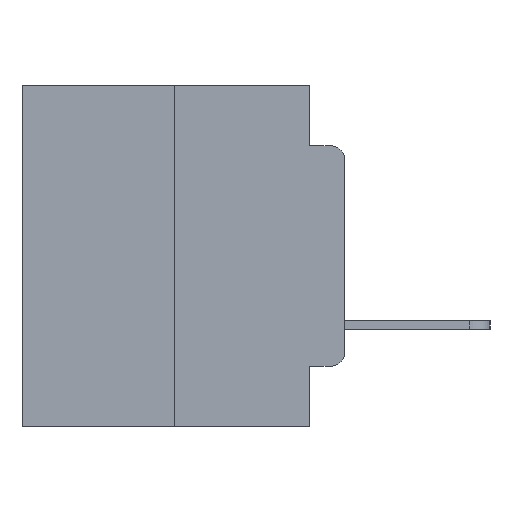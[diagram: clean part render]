
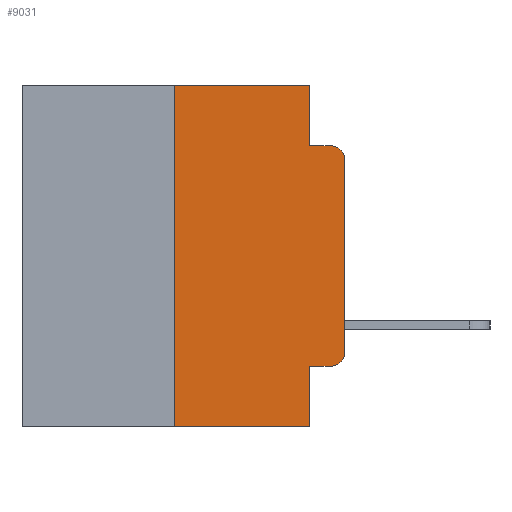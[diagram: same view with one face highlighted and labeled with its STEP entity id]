
A CAD part, left-side view. The second image highlights one B-rep face of the part: STEP entity #9031.
In plain terms, the highlighted planar face has unit normal (-1, 0, 0).
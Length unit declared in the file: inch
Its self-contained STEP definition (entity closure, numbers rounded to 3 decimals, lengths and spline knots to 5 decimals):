
#978 = DIRECTION ( 'NONE',  ( 1., 0., 0. ) ) ;
#1343 = ORIENTED_EDGE ( 'NONE', *, *, #14991, .T. ) ;
#1379 = ORIENTED_EDGE ( 'NONE', *, *, #8385, .F. ) ;
#1432 = ORIENTED_EDGE ( 'NONE', *, *, #3981, .F. ) ;
#1718 = CARTESIAN_POINT ( 'NONE',  ( 0., 0.473, 0. ) ) ;
#2085 = LINE ( 'NONE', #13930, #7773 ) ;
#2167 = PLANE ( 'NONE',  #11923 ) ;
#3199 = ORIENTED_EDGE ( 'NONE', *, *, #7303, .T. ) ;
#3981 = EDGE_CURVE ( 'NONE', #24997, #15552, #4936, .T. ) ;
#4006 = CARTESIAN_POINT ( 'NONE',  ( 0., 0.051, -0.0885 ) ) ;
#4120 = CARTESIAN_POINT ( 'NONE',  ( 0., 0.473, -0.5 ) ) ;
#4145 = CIRCLE ( 'NONE', #16932, 0.02 ) ;
#4783 = ORIENTED_EDGE ( 'NONE', *, *, #8187, .F. ) ;
#4809 = DIRECTION ( 'NONE',  ( 0., 0., -1. ) ) ;
#4936 = LINE ( 'NONE', #8817, #14816 ) ;
#5304 = VECTOR ( 'NONE', #20444, 39.37008 ) ;
#5547 = VERTEX_POINT ( 'NONE', #21693 ) ;
#5571 = FACE_OUTER_BOUND ( 'NONE', #15620, .T. ) ;
#5613 = VERTEX_POINT ( 'NONE', #19469 ) ;
#5883 = CARTESIAN_POINT ( 'NONE',  ( 0., 0., -0.1085 ) ) ;
#6039 = VECTOR ( 'NONE', #6686, 39.37008 ) ;
#6062 = VECTOR ( 'NONE', #9578, 39.37008 ) ;
#6412 = ORIENTED_EDGE ( 'NONE', *, *, #8388, .T. ) ;
#6423 = DIRECTION ( 'NONE',  ( 0., 0., -1. ) ) ;
#6652 = DIRECTION ( 'NONE',  ( 0., -1., 0. ) ) ;
#6680 = DIRECTION ( 'NONE',  ( -1., 0., 0. ) ) ;
#6686 = DIRECTION ( 'NONE',  ( 0., 0., -1. ) ) ;
#6707 = CARTESIAN_POINT ( 'NONE',  ( 0., 0.051, -0.4115 ) ) ;
#6713 = LINE ( 'NONE', #6707, #26224 ) ;
#6737 = CARTESIAN_POINT ( 'NONE',  ( 0., 0.051, 0. ) ) ;
#6741 = CARTESIAN_POINT ( 'NONE',  ( 0., 0.02, -0.1085 ) ) ;
#7303 = EDGE_CURVE ( 'NONE', #12543, #11504, #21738, .T. ) ;
#7340 = EDGE_CURVE ( 'NONE', #11504, #5547, #4145, .T. ) ;
#7463 = EDGE_CURVE ( 'NONE', #13498, #5547, #12701, .T. ) ;
#7526 = ORIENTED_EDGE ( 'NONE', *, *, #8641, .T. ) ;
#7773 = VECTOR ( 'NONE', #14446, 39.37008 ) ;
#8112 = EDGE_CURVE ( 'NONE', #15552, #13498, #2085, .T. ) ;
#8187 = EDGE_CURVE ( 'NONE', #5613, #24997, #16811, .T. ) ;
#8385 = EDGE_CURVE ( 'NONE', #17269, #15461, #22303, .T. ) ;
#8388 = EDGE_CURVE ( 'NONE', #17269, #11099, #6713, .T. ) ;
#8641 = EDGE_CURVE ( 'NONE', #11099, #12543, #20171, .T. ) ;
#8817 = CARTESIAN_POINT ( 'NONE',  ( 0., 0.473, 0. ) ) ;
#9031 = ADVANCED_FACE ( 'NONE', ( #5571 ), #2167, .F. ) ;
#9181 = CARTESIAN_POINT ( 'NONE',  ( 0., 0.051, -0.4115 ) ) ;
#9578 = DIRECTION ( 'NONE',  ( 0., 0., 1. ) ) ;
#9769 = CARTESIAN_POINT ( 'NONE',  ( 0., 0., 0. ) ) ;
#11099 = VERTEX_POINT ( 'NONE', #19550 ) ;
#11504 = VERTEX_POINT ( 'NONE', #5883 ) ;
#11923 = AXIS2_PLACEMENT_3D ( 'NONE', #1718, #978, #12239 ) ;
#12067 = VECTOR ( 'NONE', #12161, 39.37008 ) ;
#12161 = DIRECTION ( 'NONE',  ( 0., 0., 1. ) ) ;
#12193 = CARTESIAN_POINT ( 'NONE',  ( 0., 0.25, 0. ) ) ;
#12239 = DIRECTION ( 'NONE',  ( 0., 0., -1. ) ) ;
#12543 = VERTEX_POINT ( 'NONE', #19851 ) ;
#12701 = LINE ( 'NONE', #26269, #17400 ) ;
#13498 = VERTEX_POINT ( 'NONE', #4006 ) ;
#13930 = CARTESIAN_POINT ( 'NONE',  ( 0., 0.051, 0. ) ) ;
#14123 = CARTESIAN_POINT ( 'NONE',  ( 0., 0.051, 0. ) ) ;
#14446 = DIRECTION ( 'NONE',  ( 0., 0., -1. ) ) ;
#14816 = VECTOR ( 'NONE', #23032, 39.37008 ) ;
#14991 = EDGE_CURVE ( 'NONE', #5613, #15461, #16427, .T. ) ;
#15461 = VERTEX_POINT ( 'NONE', #23623 ) ;
#15552 = VERTEX_POINT ( 'NONE', #14123 ) ;
#15620 = EDGE_LOOP ( 'NONE', ( #3199, #19325, #25422, #26311, #1432, #4783, #1343, #1379, #6412, #7526 ) ) ;
#16427 = LINE ( 'NONE', #4120, #5304 ) ;
#16811 = LINE ( 'NONE', #12193, #12067 ) ;
#16932 = AXIS2_PLACEMENT_3D ( 'NONE', #6741, #6680, #6423 ) ;
#17269 = VERTEX_POINT ( 'NONE', #9181 ) ;
#17400 = VECTOR ( 'NONE', #26222, 39.37008 ) ;
#17450 = AXIS2_PLACEMENT_3D ( 'NONE', #23006, #23091, #4809 ) ;
#19325 = ORIENTED_EDGE ( 'NONE', *, *, #7340, .T. ) ;
#19469 = CARTESIAN_POINT ( 'NONE',  ( 0., 0.25, -0.5 ) ) ;
#19550 = CARTESIAN_POINT ( 'NONE',  ( 0., 0.02, -0.4115 ) ) ;
#19851 = CARTESIAN_POINT ( 'NONE',  ( 0., 0., -0.3915 ) ) ;
#20171 = CIRCLE ( 'NONE', #17450, 0.02 ) ;
#20444 = DIRECTION ( 'NONE',  ( 0., -1., 0. ) ) ;
#21693 = CARTESIAN_POINT ( 'NONE',  ( 0., 0.02, -0.0885 ) ) ;
#21738 = LINE ( 'NONE', #9769, #6062 ) ;
#22303 = LINE ( 'NONE', #6737, #6039 ) ;
#23006 = CARTESIAN_POINT ( 'NONE',  ( 0., 0.02, -0.3915 ) ) ;
#23032 = DIRECTION ( 'NONE',  ( 0., -1., 0. ) ) ;
#23091 = DIRECTION ( 'NONE',  ( -1., 0., 0. ) ) ;
#23623 = CARTESIAN_POINT ( 'NONE',  ( 0., 0.051, -0.5 ) ) ;
#24564 = CARTESIAN_POINT ( 'NONE',  ( 0., 0.25, 0. ) ) ;
#24997 = VERTEX_POINT ( 'NONE', #24564 ) ;
#25422 = ORIENTED_EDGE ( 'NONE', *, *, #7463, .F. ) ;
#26222 = DIRECTION ( 'NONE',  ( 0., -1., 0. ) ) ;
#26224 = VECTOR ( 'NONE', #6652, 39.37008 ) ;
#26269 = CARTESIAN_POINT ( 'NONE',  ( 0., 0.051, -0.0885 ) ) ;
#26311 = ORIENTED_EDGE ( 'NONE', *, *, #8112, .F. ) ;
